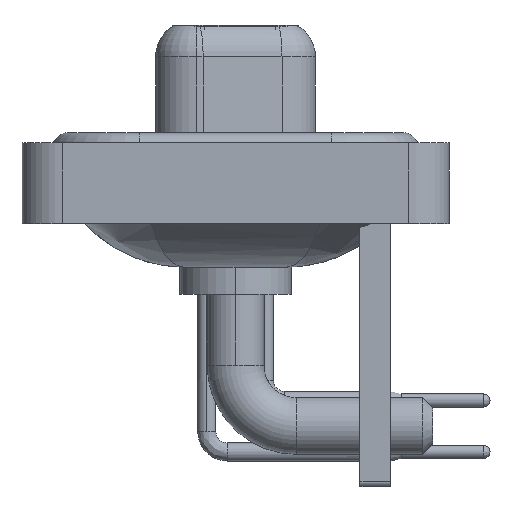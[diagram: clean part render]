
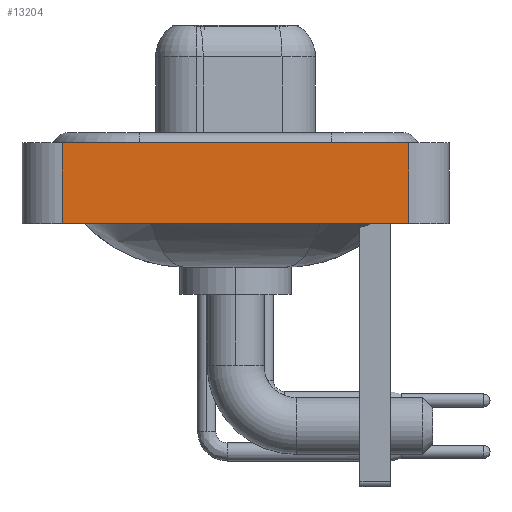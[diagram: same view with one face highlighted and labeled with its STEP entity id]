
A CAD part, left-side view. The second image highlights one B-rep face of the part: STEP entity #13204.
In plain terms, the highlighted planar face has unit normal (-1, 0, 0).
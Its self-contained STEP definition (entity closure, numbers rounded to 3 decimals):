
#482 = VECTOR ( 'NONE', #18231, 1000. ) ;
#564 = LINE ( 'NONE', #7510, #3619 ) ;
#1148 = LINE ( 'NONE', #7774, #6335 ) ;
#1456 = LINE ( 'NONE', #15910, #13140 ) ;
#2366 = EDGE_CURVE ( 'NONE', #3074, #17039, #1456, .T. ) ;
#2786 = CARTESIAN_POINT ( 'NONE',  ( -7.3, -8.55, 0.4 ) ) ;
#3074 = VERTEX_POINT ( 'NONE', #21077 ) ;
#3122 = AXIS2_PLACEMENT_3D ( 'NONE', #16584, #21144, #3383 ) ;
#3383 = DIRECTION ( 'NONE',  ( 0., 0., 1. ) ) ;
#3619 = VECTOR ( 'NONE', #14125, 1000. ) ;
#4527 = DIRECTION ( 'NONE',  ( 0., -1., 0. ) ) ;
#5006 = LINE ( 'NONE', #13480, #482 ) ;
#5937 = ORIENTED_EDGE ( 'NONE', *, *, #19033, .T. ) ;
#6271 = VERTEX_POINT ( 'NONE', #18059 ) ;
#6335 = VECTOR ( 'NONE', #9397, 1000. ) ;
#7510 = CARTESIAN_POINT ( 'NONE',  ( -7.3, -8.55, -3.6 ) ) ;
#7774 = CARTESIAN_POINT ( 'NONE',  ( -7.3, -8.55, 0.4 ) ) ;
#8351 = EDGE_CURVE ( 'NONE', #6271, #13594, #1148, .T. ) ;
#9397 = DIRECTION ( 'NONE',  ( 0., -1., 0. ) ) ;
#10414 = ORIENTED_EDGE ( 'NONE', *, *, #19958, .F. ) ;
#12899 = PLANE ( 'NONE',  #3122 ) ;
#13140 = VECTOR ( 'NONE', #4527, 1000. ) ;
#13204 = ADVANCED_FACE ( 'NONE', ( #14963 ), #12899, .T. ) ;
#13480 = CARTESIAN_POINT ( 'NONE',  ( -7.3, 8.55, -3.6 ) ) ;
#13534 = ORIENTED_EDGE ( 'NONE', *, *, #2366, .T. ) ;
#13594 = VERTEX_POINT ( 'NONE', #2786 ) ;
#14125 = DIRECTION ( 'NONE',  ( 0., 0., 1. ) ) ;
#14827 = CARTESIAN_POINT ( 'NONE',  ( -7.3, -8.55, -3.6 ) ) ;
#14963 = FACE_OUTER_BOUND ( 'NONE', #18160, .T. ) ;
#15910 = CARTESIAN_POINT ( 'NONE',  ( -7.3, -8.55, -3.6 ) ) ;
#16398 = ORIENTED_EDGE ( 'NONE', *, *, #8351, .F. ) ;
#16584 = CARTESIAN_POINT ( 'NONE',  ( -7.3, -8.55, -3.6 ) ) ;
#17039 = VERTEX_POINT ( 'NONE', #14827 ) ;
#18059 = CARTESIAN_POINT ( 'NONE',  ( -7.3, 8.55, 0.4 ) ) ;
#18160 = EDGE_LOOP ( 'NONE', ( #5937, #16398, #10414, #13534 ) ) ;
#18231 = DIRECTION ( 'NONE',  ( 0., 0., 1. ) ) ;
#19033 = EDGE_CURVE ( 'NONE', #17039, #13594, #564, .T. ) ;
#19958 = EDGE_CURVE ( 'NONE', #3074, #6271, #5006, .T. ) ;
#21077 = CARTESIAN_POINT ( 'NONE',  ( -7.3, 8.55, -3.6 ) ) ;
#21144 = DIRECTION ( 'NONE',  ( -1., 0., 0. ) ) ;
